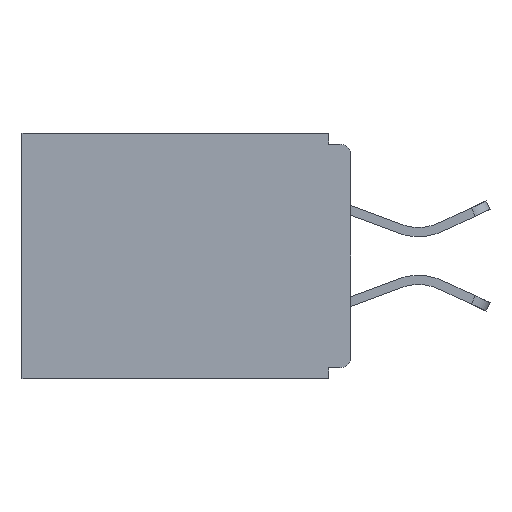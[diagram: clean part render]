
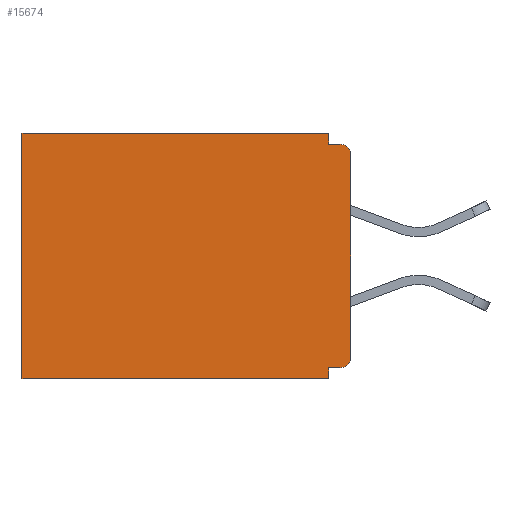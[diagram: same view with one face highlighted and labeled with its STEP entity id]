
A CAD part, left-side view. The second image highlights one B-rep face of the part: STEP entity #15674.
In plain terms, the highlighted planar face has unit normal (-1, 0, 0).
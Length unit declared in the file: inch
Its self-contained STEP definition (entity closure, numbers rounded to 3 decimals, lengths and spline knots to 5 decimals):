
#169 = EDGE_CURVE ( 'NONE', #18108, #22337, #14420, .T. ) ;
#1014 = CARTESIAN_POINT ( 'NONE',  ( 0.298, 0., 0. ) ) ;
#1172 = EDGE_CURVE ( 'NONE', #11205, #20828, #17566, .T. ) ;
#1496 = CARTESIAN_POINT ( 'NONE',  ( 0.298, 0., 0. ) ) ;
#1795 = CARTESIAN_POINT ( 'NONE',  ( 0.298, 0.031, -0.343 ) ) ;
#2120 = CARTESIAN_POINT ( 'NONE',  ( 0.298, 0.46, 0. ) ) ;
#2611 = ORIENTED_EDGE ( 'NONE', *, *, #5222, .F. ) ;
#3243 = CARTESIAN_POINT ( 'NONE',  ( 0.298, 0., -0.328 ) ) ;
#3598 = DIRECTION ( 'NONE',  ( 0., 1., 0. ) ) ;
#3602 = CARTESIAN_POINT ( 'NONE',  ( 0.298, 0.015, -0.328 ) ) ;
#4195 = CARTESIAN_POINT ( 'NONE',  ( 0.298, 0.031, -0.343 ) ) ;
#4357 = LINE ( 'NONE', #14900, #11929 ) ;
#4619 = VECTOR ( 'NONE', #10501, 39.37008 ) ;
#5188 = EDGE_CURVE ( 'NONE', #11205, #22337, #21374, .T. ) ;
#5210 = CARTESIAN_POINT ( 'NONE',  ( 0.298, 0.015, -0.313 ) ) ;
#5222 = EDGE_CURVE ( 'NONE', #5832, #12882, #19818, .T. ) ;
#5345 = VECTOR ( 'NONE', #24173, 39.37008 ) ;
#5444 = ORIENTED_EDGE ( 'NONE', *, *, #24577, .F. ) ;
#5696 = VECTOR ( 'NONE', #3598, 39.37008 ) ;
#5796 = CARTESIAN_POINT ( 'NONE',  ( 0.298, 0.46, 0. ) ) ;
#5832 = VERTEX_POINT ( 'NONE', #4195 ) ;
#6250 = ORIENTED_EDGE ( 'NONE', *, *, #10022, .T. ) ;
#6301 = AXIS2_PLACEMENT_3D ( 'NONE', #22468, #24478, #6351 ) ;
#6351 = DIRECTION ( 'NONE',  ( 0., 0., -1. ) ) ;
#6530 = ORIENTED_EDGE ( 'NONE', *, *, #5188, .F. ) ;
#7367 = CARTESIAN_POINT ( 'NONE',  ( 0.298, 0., -0.03 ) ) ;
#7717 = DIRECTION ( 'NONE',  ( 0., 1., 0. ) ) ;
#10022 = EDGE_CURVE ( 'NONE', #19853, #12882, #24882, .T. ) ;
#10501 = DIRECTION ( 'NONE',  ( 0., 0., -1. ) ) ;
#10612 = VECTOR ( 'NONE', #11223, 39.37008 ) ;
#11205 = VERTEX_POINT ( 'NONE', #7367 ) ;
#11223 = DIRECTION ( 'NONE',  ( 0., 0., -1. ) ) ;
#11329 = ORIENTED_EDGE ( 'NONE', *, *, #169, .T. ) ;
#11929 = VECTOR ( 'NONE', #16941, 39.37008 ) ;
#12016 = EDGE_LOOP ( 'NONE', ( #16145, #12797, #5444, #19251, #6250, #2611, #19207, #15390, #11329, #6530 ) ) ;
#12533 = CARTESIAN_POINT ( 'NONE',  ( 0.298, 0.031, -0.015 ) ) ;
#12797 = ORIENTED_EDGE ( 'NONE', *, *, #16019, .F. ) ;
#12882 = VERTEX_POINT ( 'NONE', #16357 ) ;
#13209 = DIRECTION ( 'NONE',  ( 1., 0., 0. ) ) ;
#13924 = CARTESIAN_POINT ( 'NONE',  ( 0.298, 0., -0.015 ) ) ;
#14103 = VECTOR ( 'NONE', #23698, 39.37008 ) ;
#14284 = AXIS2_PLACEMENT_3D ( 'NONE', #5210, #15308, #21653 ) ;
#14420 = CIRCLE ( 'NONE', #14284, 0.015 ) ;
#14900 = CARTESIAN_POINT ( 'NONE',  ( 0.298, 0.031, -0.343 ) ) ;
#15140 = CARTESIAN_POINT ( 'NONE',  ( 0.298, 0., -0.343 ) ) ;
#15308 = DIRECTION ( 'NONE',  ( -1., 0., 0. ) ) ;
#15353 = CARTESIAN_POINT ( 'NONE',  ( 0.298, 0., 0. ) ) ;
#15390 = ORIENTED_EDGE ( 'NONE', *, *, #25096, .F. ) ;
#15583 = VERTEX_POINT ( 'NONE', #20239 ) ;
#15674 = ADVANCED_FACE ( 'NONE', ( #25285 ), #23032, .F. ) ;
#16019 = EDGE_CURVE ( 'NONE', #25634, #20828, #18023, .T. ) ;
#16119 = DIRECTION ( 'NONE',  ( 0., 0., -1. ) ) ;
#16145 = ORIENTED_EDGE ( 'NONE', *, *, #1172, .T. ) ;
#16357 = CARTESIAN_POINT ( 'NONE',  ( 0.298, 0.46, -0.343 ) ) ;
#16941 = DIRECTION ( 'NONE',  ( 0., 0., -1. ) ) ;
#17124 = AXIS2_PLACEMENT_3D ( 'NONE', #15353, #13209, #23307 ) ;
#17566 = CIRCLE ( 'NONE', #6301, 0.015 ) ;
#17891 = CARTESIAN_POINT ( 'NONE',  ( 0.298, 0.031, 0. ) ) ;
#18023 = LINE ( 'NONE', #13924, #5345 ) ;
#18108 = VERTEX_POINT ( 'NONE', #3602 ) ;
#18816 = CARTESIAN_POINT ( 'NONE',  ( 0.298, 0., -0.313 ) ) ;
#19207 = ORIENTED_EDGE ( 'NONE', *, *, #20223, .F. ) ;
#19251 = ORIENTED_EDGE ( 'NONE', *, *, #23160, .T. ) ;
#19703 = LINE ( 'NONE', #1795, #23813 ) ;
#19818 = LINE ( 'NONE', #15140, #14103 ) ;
#19853 = VERTEX_POINT ( 'NONE', #5796 ) ;
#20223 = EDGE_CURVE ( 'NONE', #15583, #5832, #19703, .T. ) ;
#20239 = CARTESIAN_POINT ( 'NONE',  ( 0.298, 0.031, -0.328 ) ) ;
#20828 = VERTEX_POINT ( 'NONE', #22078 ) ;
#21374 = LINE ( 'NONE', #1014, #10612 ) ;
#21653 = DIRECTION ( 'NONE',  ( 0., 0., -1. ) ) ;
#22078 = CARTESIAN_POINT ( 'NONE',  ( 0.298, 0.015, -0.015 ) ) ;
#22337 = VERTEX_POINT ( 'NONE', #18816 ) ;
#22377 = LINE ( 'NONE', #3243, #25861 ) ;
#22468 = CARTESIAN_POINT ( 'NONE',  ( 0.298, 0.015, -0.03 ) ) ;
#23032 = PLANE ( 'NONE',  #17124 ) ;
#23160 = EDGE_CURVE ( 'NONE', #24889, #19853, #24371, .T. ) ;
#23307 = DIRECTION ( 'NONE',  ( 0., 0., -1. ) ) ;
#23698 = DIRECTION ( 'NONE',  ( 0., 1., 0. ) ) ;
#23813 = VECTOR ( 'NONE', #16119, 39.37008 ) ;
#24173 = DIRECTION ( 'NONE',  ( 0., -1., 0. ) ) ;
#24371 = LINE ( 'NONE', #1496, #5696 ) ;
#24478 = DIRECTION ( 'NONE',  ( -1., 0., 0. ) ) ;
#24577 = EDGE_CURVE ( 'NONE', #24889, #25634, #4357, .T. ) ;
#24882 = LINE ( 'NONE', #2120, #4619 ) ;
#24889 = VERTEX_POINT ( 'NONE', #17891 ) ;
#25096 = EDGE_CURVE ( 'NONE', #18108, #15583, #22377, .T. ) ;
#25285 = FACE_OUTER_BOUND ( 'NONE', #12016, .T. ) ;
#25634 = VERTEX_POINT ( 'NONE', #12533 ) ;
#25861 = VECTOR ( 'NONE', #7717, 39.37008 ) ;
